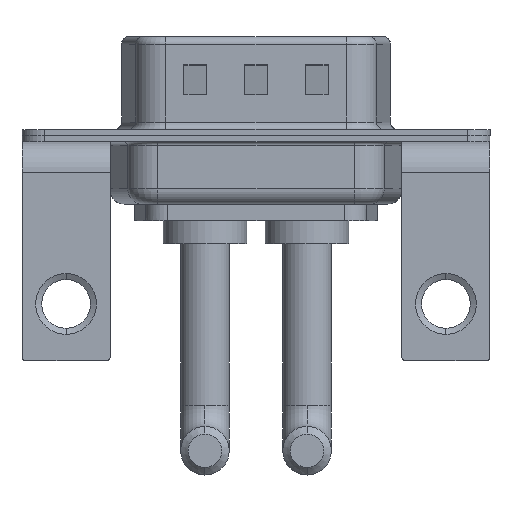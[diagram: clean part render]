
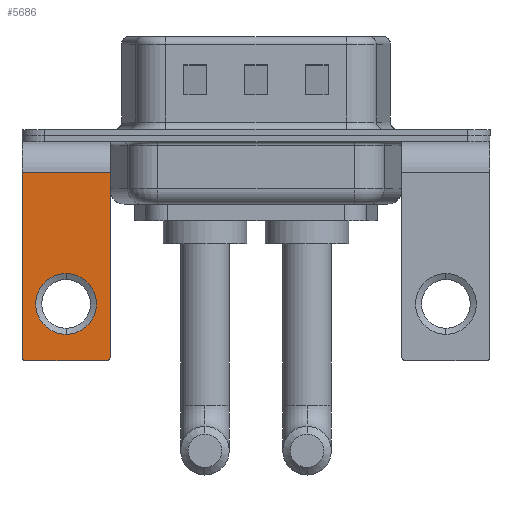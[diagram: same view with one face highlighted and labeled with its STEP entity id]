
A CAD part, front view. The second image highlights one B-rep face of the part: STEP entity #5686.
In plain terms, the highlighted planar face has unit normal (0, -1, 0).
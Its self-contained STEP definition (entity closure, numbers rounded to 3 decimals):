
#93 = CARTESIAN_POINT ( 'NONE',  ( 2.9, -6.25, -2.4 ) ) ;
#170 = ORIENTED_EDGE ( 'NONE', *, *, #2157, .T. ) ;
#303 = DIRECTION ( 'NONE',  ( 0., 0., 1. ) ) ;
#313 = AXIS2_PLACEMENT_3D ( 'NONE', #431, #11053, #1731 ) ;
#431 = CARTESIAN_POINT ( 'NONE',  ( 0., -6.25, -11.07 ) ) ;
#775 = VERTEX_POINT ( 'NONE', #3615 ) ;
#970 = AXIS2_PLACEMENT_3D ( 'NONE', #8831, #13492, #3102 ) ;
#1537 = CIRCLE ( 'NONE', #313, 2. ) ;
#1731 = DIRECTION ( 'NONE',  ( 0., 0., 1. ) ) ;
#1943 = ORIENTED_EDGE ( 'NONE', *, *, #9201, .T. ) ;
#2129 = ORIENTED_EDGE ( 'NONE', *, *, #6594, .T. ) ;
#2157 = EDGE_CURVE ( 'NONE', #12381, #13321, #1537, .T. ) ;
#2287 = EDGE_CURVE ( 'NONE', #9324, #7575, #9829, .T. ) ;
#2367 = FACE_BOUND ( 'NONE', #4457, .T. ) ;
#2413 = CARTESIAN_POINT ( 'NONE',  ( 2.9, -6.25, -14.55 ) ) ;
#2414 = ORIENTED_EDGE ( 'NONE', *, *, #2287, .T. ) ;
#2473 = EDGE_CURVE ( 'NONE', #13321, #12381, #14228, .T. ) ;
#2815 = CARTESIAN_POINT ( 'NONE',  ( 0., -6.25, -9.07 ) ) ;
#3102 = DIRECTION ( 'NONE',  ( 0., 0., 1. ) ) ;
#3282 = CARTESIAN_POINT ( 'NONE',  ( -2.9, -6.25, -14.55 ) ) ;
#3615 = CARTESIAN_POINT ( 'NONE',  ( 2.9, -6.25, -2.4 ) ) ;
#3735 = FACE_OUTER_BOUND ( 'NONE', #3742, .T. ) ;
#3742 = EDGE_LOOP ( 'NONE', ( #1943, #2414, #14173, #2129, #8779, #10632 ) ) ;
#3911 = VECTOR ( 'NONE', #5882, 1000. ) ;
#4455 = CARTESIAN_POINT ( 'NONE',  ( -2.9, -6.25, -2.4 ) ) ;
#4457 = EDGE_LOOP ( 'NONE', ( #170, #9427 ) ) ;
#4549 = DIRECTION ( 'NONE',  ( 0., 1., 0. ) ) ;
#4608 = LINE ( 'NONE', #93, #3911 ) ;
#4657 = VERTEX_POINT ( 'NONE', #5881 ) ;
#4742 = PLANE ( 'NONE',  #9229 ) ;
#5082 = CARTESIAN_POINT ( 'NONE',  ( -2.65, -6.25, -14.55 ) ) ;
#5121 = CARTESIAN_POINT ( 'NONE',  ( -2.9, -6.25, -2.4 ) ) ;
#5686 = ADVANCED_FACE ( 'NONE', ( #2367, #3735 ), #4742, .F. ) ;
#5881 = CARTESIAN_POINT ( 'NONE',  ( 2.65, -6.25, -14.8 ) ) ;
#5882 = DIRECTION ( 'NONE',  ( 0., 0., -1. ) ) ;
#5934 = AXIS2_PLACEMENT_3D ( 'NONE', #7834, #4549, #11490 ) ;
#6200 = EDGE_CURVE ( 'NONE', #4657, #7575, #9438, .T. ) ;
#6594 = EDGE_CURVE ( 'NONE', #4657, #13549, #10714, .T. ) ;
#7121 = EDGE_CURVE ( 'NONE', #775, #13549, #4608, .T. ) ;
#7575 = VERTEX_POINT ( 'NONE', #12618 ) ;
#7640 = AXIS2_PLACEMENT_3D ( 'NONE', #5082, #13189, #14410 ) ;
#7811 = CARTESIAN_POINT ( 'NONE',  ( 0., -6.25, -13.07 ) ) ;
#7834 = CARTESIAN_POINT ( 'NONE',  ( 0., -6.25, -11.07 ) ) ;
#7894 = VERTEX_POINT ( 'NONE', #4455 ) ;
#8065 = DIRECTION ( 'NONE',  ( -1., 0., 0. ) ) ;
#8388 = CARTESIAN_POINT ( 'NONE',  ( 2.9, -6.25, -2.4 ) ) ;
#8779 = ORIENTED_EDGE ( 'NONE', *, *, #7121, .F. ) ;
#8831 = CARTESIAN_POINT ( 'NONE',  ( 2.65, -6.25, -14.55 ) ) ;
#9008 = CARTESIAN_POINT ( 'NONE',  ( 2.9, -6.25, -2.4 ) ) ;
#9201 = EDGE_CURVE ( 'NONE', #7894, #9324, #14222, .T. ) ;
#9229 = AXIS2_PLACEMENT_3D ( 'NONE', #8388, #13065, #303 ) ;
#9324 = VERTEX_POINT ( 'NONE', #3282 ) ;
#9427 = ORIENTED_EDGE ( 'NONE', *, *, #2473, .T. ) ;
#9438 = LINE ( 'NONE', #13885, #11449 ) ;
#9829 = CIRCLE ( 'NONE', #7640, 0.25 ) ;
#10632 = ORIENTED_EDGE ( 'NONE', *, *, #10883, .T. ) ;
#10714 = CIRCLE ( 'NONE', #970, 0.25 ) ;
#10784 = DIRECTION ( 'NONE',  ( 0., 0., -1. ) ) ;
#10883 = EDGE_CURVE ( 'NONE', #775, #7894, #13600, .T. ) ;
#11053 = DIRECTION ( 'NONE',  ( 0., 1., 0. ) ) ;
#11063 = VECTOR ( 'NONE', #12389, 1000. ) ;
#11449 = VECTOR ( 'NONE', #8065, 1000. ) ;
#11490 = DIRECTION ( 'NONE',  ( 0., 0., 1. ) ) ;
#12381 = VERTEX_POINT ( 'NONE', #7811 ) ;
#12389 = DIRECTION ( 'NONE',  ( -1., 0., 0. ) ) ;
#12618 = CARTESIAN_POINT ( 'NONE',  ( -2.65, -6.25, -14.8 ) ) ;
#13065 = DIRECTION ( 'NONE',  ( 0., 1., 0. ) ) ;
#13189 = DIRECTION ( 'NONE',  ( 0., -1., 0. ) ) ;
#13321 = VERTEX_POINT ( 'NONE', #2815 ) ;
#13492 = DIRECTION ( 'NONE',  ( 0., -1., 0. ) ) ;
#13549 = VERTEX_POINT ( 'NONE', #2413 ) ;
#13600 = LINE ( 'NONE', #9008, #11063 ) ;
#13885 = CARTESIAN_POINT ( 'NONE',  ( 2.9, -6.25, -14.8 ) ) ;
#14070 = VECTOR ( 'NONE', #10784, 1000. ) ;
#14173 = ORIENTED_EDGE ( 'NONE', *, *, #6200, .F. ) ;
#14222 = LINE ( 'NONE', #5121, #14070 ) ;
#14228 = CIRCLE ( 'NONE', #5934, 2. ) ;
#14410 = DIRECTION ( 'NONE',  ( 0., 0., 1. ) ) ;
